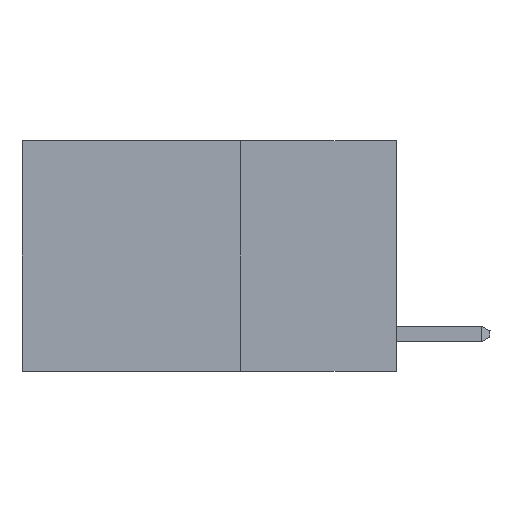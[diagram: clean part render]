
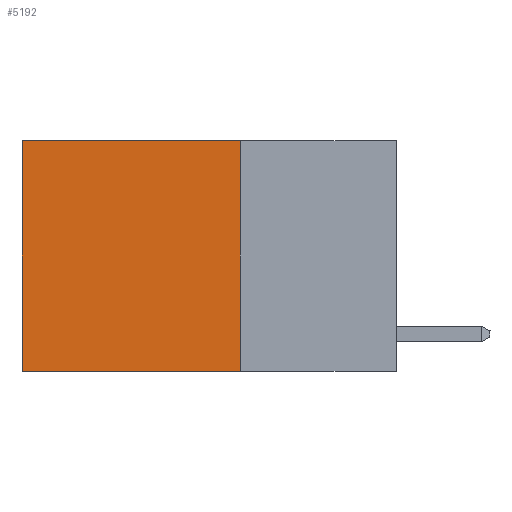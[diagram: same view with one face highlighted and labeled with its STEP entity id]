
A CAD part, left-side view. The second image highlights one B-rep face of the part: STEP entity #5192.
In plain terms, the highlighted planar face has unit normal (-1, 0, 0).
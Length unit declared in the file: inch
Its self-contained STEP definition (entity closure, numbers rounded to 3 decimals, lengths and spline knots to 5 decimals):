
#980 = ORIENTED_EDGE ( 'NONE', *, *, #23663, .F. ) ;
#1067 = DIRECTION ( 'NONE',  ( 0., 1., 0. ) ) ;
#1108 = CARTESIAN_POINT ( 'NONE',  ( 0.2625, 0.6, -0.37 ) ) ;
#1336 = CARTESIAN_POINT ( 'NONE',  ( 0.2625, 0.25, 0. ) ) ;
#2077 = CARTESIAN_POINT ( 'NONE',  ( 0.2625, 0.25, 0. ) ) ;
#3029 = ORIENTED_EDGE ( 'NONE', *, *, #14976, .T. ) ;
#3380 = DIRECTION ( 'NONE',  ( 0., 0., -1. ) ) ;
#3790 = VERTEX_POINT ( 'NONE', #7055 ) ;
#4384 = EDGE_CURVE ( 'NONE', #3790, #22976, #15192, .T. ) ;
#5192 = ADVANCED_FACE ( 'NONE', ( #25145 ), #13582, .F. ) ;
#5199 = LINE ( 'NONE', #24544, #9994 ) ;
#7055 = CARTESIAN_POINT ( 'NONE',  ( 0.2625, 0.25, -0.37 ) ) ;
#7111 = CARTESIAN_POINT ( 'NONE',  ( 0.2625, 0.25, -0.37 ) ) ;
#9840 = ORIENTED_EDGE ( 'NONE', *, *, #19528, .T. ) ;
#9994 = VECTOR ( 'NONE', #16493, 39.37008 ) ;
#10838 = LINE ( 'NONE', #25861, #15578 ) ;
#12107 = ORIENTED_EDGE ( 'NONE', *, *, #4384, .F. ) ;
#13582 = PLANE ( 'NONE',  #15064 ) ;
#14976 = EDGE_CURVE ( 'NONE', #25582, #22976, #5199, .T. ) ;
#14986 = CARTESIAN_POINT ( 'NONE',  ( 0.2625, 0.25, 0. ) ) ;
#15064 = AXIS2_PLACEMENT_3D ( 'NONE', #1336, #15582, #3380 ) ;
#15192 = LINE ( 'NONE', #7111, #19915 ) ;
#15578 = VECTOR ( 'NONE', #21787, 39.37008 ) ;
#15582 = DIRECTION ( 'NONE',  ( 1., 0., 0. ) ) ;
#16493 = DIRECTION ( 'NONE',  ( 0., 0., -1. ) ) ;
#17011 = DIRECTION ( 'NONE',  ( 0., 1., 0. ) ) ;
#18009 = VERTEX_POINT ( 'NONE', #2077 ) ;
#18074 = EDGE_LOOP ( 'NONE', ( #3029, #12107, #980, #9840 ) ) ;
#19234 = LINE ( 'NONE', #14986, #24005 ) ;
#19528 = EDGE_CURVE ( 'NONE', #18009, #25582, #19234, .T. ) ;
#19915 = VECTOR ( 'NONE', #1067, 39.37008 ) ;
#21787 = DIRECTION ( 'NONE',  ( 0., 0., -1. ) ) ;
#22976 = VERTEX_POINT ( 'NONE', #1108 ) ;
#23663 = EDGE_CURVE ( 'NONE', #18009, #3790, #10838, .T. ) ;
#24005 = VECTOR ( 'NONE', #17011, 39.37008 ) ;
#24544 = CARTESIAN_POINT ( 'NONE',  ( 0.2625, 0.6, 0. ) ) ;
#25145 = FACE_OUTER_BOUND ( 'NONE', #18074, .T. ) ;
#25582 = VERTEX_POINT ( 'NONE', #25602 ) ;
#25602 = CARTESIAN_POINT ( 'NONE',  ( 0.2625, 0.6, 0. ) ) ;
#25861 = CARTESIAN_POINT ( 'NONE',  ( 0.2625, 0.25, 0. ) ) ;
